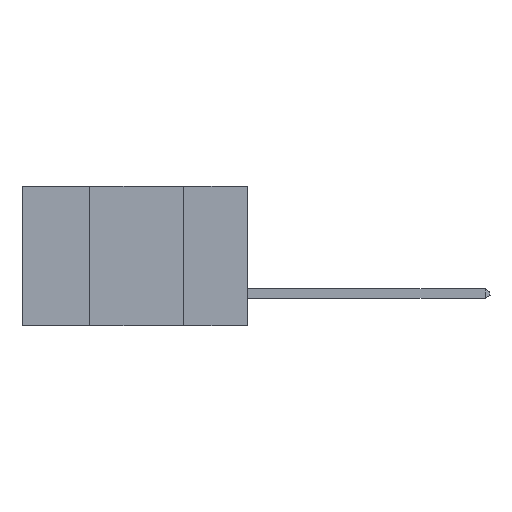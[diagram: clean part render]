
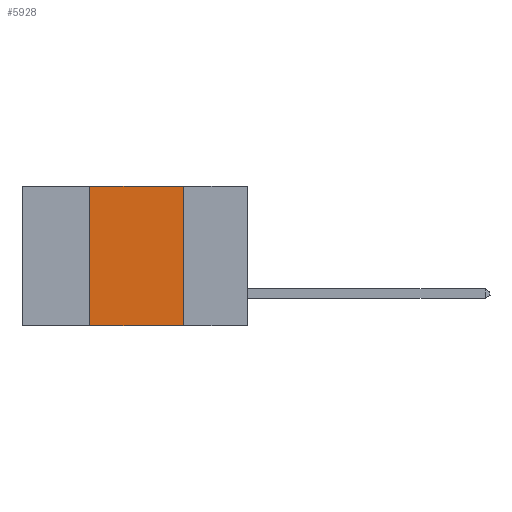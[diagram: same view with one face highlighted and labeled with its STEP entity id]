
A CAD part, left-side view. The second image highlights one B-rep face of the part: STEP entity #5928.
In plain terms, the highlighted planar face has unit normal (-1, 0, 0).
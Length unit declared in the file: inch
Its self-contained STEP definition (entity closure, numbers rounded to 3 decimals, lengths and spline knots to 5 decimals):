
#124 = PLANE ( 'NONE',  #13979 ) ;
#145 = CARTESIAN_POINT ( 'NONE',  ( 0., 0.17, 0. ) ) ;
#210 = DIRECTION ( 'NONE',  ( 0., 0., -1. ) ) ;
#327 = DIRECTION ( 'NONE',  ( 0., 0., -1. ) ) ;
#1103 = ORIENTED_EDGE ( 'NONE', *, *, #7973, .F. ) ;
#1887 = VECTOR ( 'NONE', #327, 39.37008 ) ;
#1912 = FACE_OUTER_BOUND ( 'NONE', #26730, .T. ) ;
#1940 = CARTESIAN_POINT ( 'NONE',  ( 0., 0.6, -0.37 ) ) ;
#2033 = ORIENTED_EDGE ( 'NONE', *, *, #20828, .F. ) ;
#2360 = DIRECTION ( 'NONE',  ( 1., 0., 0. ) ) ;
#4018 = CARTESIAN_POINT ( 'NONE',  ( 0., 0.17, -0.37 ) ) ;
#4215 = CARTESIAN_POINT ( 'NONE',  ( 0., 0.17, 0. ) ) ;
#5715 = LINE ( 'NONE', #145, #1887 ) ;
#5928 = ADVANCED_FACE ( 'NONE', ( #1912 ), #124, .F. ) ;
#7428 = LINE ( 'NONE', #1940, #16859 ) ;
#7973 = EDGE_CURVE ( 'NONE', #25201, #16899, #27241, .T. ) ;
#9079 = CARTESIAN_POINT ( 'NONE',  ( 0., 0.6, 0. ) ) ;
#10963 = VERTEX_POINT ( 'NONE', #4018 ) ;
#11097 = CARTESIAN_POINT ( 'NONE',  ( 0., 0.42, -0.37 ) ) ;
#12930 = EDGE_CURVE ( 'NONE', #25623, #10963, #7428, .T. ) ;
#13979 = AXIS2_PLACEMENT_3D ( 'NONE', #9079, #2360, #210 ) ;
#14109 = CARTESIAN_POINT ( 'NONE',  ( 0., 0.42, 0. ) ) ;
#14480 = EDGE_CURVE ( 'NONE', #25623, #25201, #28113, .T. ) ;
#16296 = DIRECTION ( 'NONE',  ( 0., 0., 1. ) ) ;
#16859 = VECTOR ( 'NONE', #24417, 39.37008 ) ;
#16899 = VERTEX_POINT ( 'NONE', #4215 ) ;
#16991 = VECTOR ( 'NONE', #16296, 39.37008 ) ;
#18426 = CARTESIAN_POINT ( 'NONE',  ( 0., 0.42, 0. ) ) ;
#19798 = ORIENTED_EDGE ( 'NONE', *, *, #12930, .T. ) ;
#20494 = CARTESIAN_POINT ( 'NONE',  ( 0., 0.6, 0. ) ) ;
#20828 = EDGE_CURVE ( 'NONE', #16899, #10963, #5715, .T. ) ;
#22360 = DIRECTION ( 'NONE',  ( 0., -1., 0. ) ) ;
#24417 = DIRECTION ( 'NONE',  ( 0., -1., 0. ) ) ;
#25145 = VECTOR ( 'NONE', #22360, 39.37008 ) ;
#25201 = VERTEX_POINT ( 'NONE', #14109 ) ;
#25623 = VERTEX_POINT ( 'NONE', #11097 ) ;
#26730 = EDGE_LOOP ( 'NONE', ( #2033, #1103, #28397, #19798 ) ) ;
#27241 = LINE ( 'NONE', #20494, #25145 ) ;
#28113 = LINE ( 'NONE', #18426, #16991 ) ;
#28397 = ORIENTED_EDGE ( 'NONE', *, *, #14480, .F. ) ;
